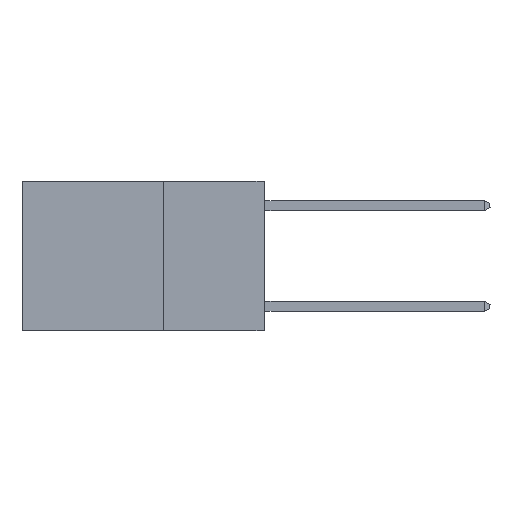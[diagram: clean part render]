
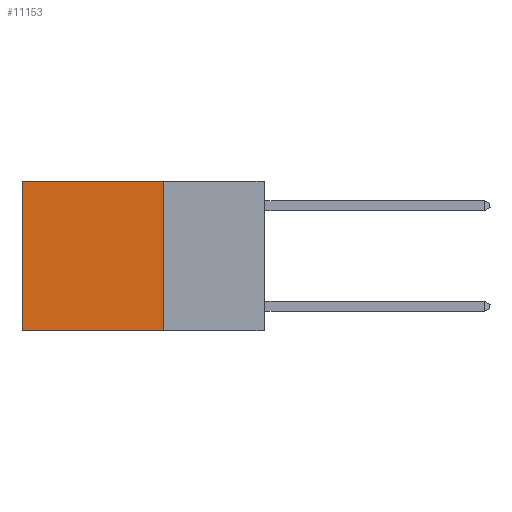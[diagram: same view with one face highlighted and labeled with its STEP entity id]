
A CAD part, left-side view. The second image highlights one B-rep face of the part: STEP entity #11153.
In plain terms, the highlighted planar face has unit normal (-1, 0, 0).
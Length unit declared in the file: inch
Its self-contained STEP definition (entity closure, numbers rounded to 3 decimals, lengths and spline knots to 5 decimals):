
#122 = CARTESIAN_POINT ( 'NONE',  ( 0.2625, 0.6, 0. ) ) ;
#252 = CARTESIAN_POINT ( 'NONE',  ( 0.2625, 0.25, -0.37 ) ) ;
#350 = EDGE_CURVE ( 'NONE', #2271, #13154, #4573, .T. ) ;
#555 = CARTESIAN_POINT ( 'NONE',  ( 0.2625, 0.25, 0. ) ) ;
#783 = ORIENTED_EDGE ( 'NONE', *, *, #350, .F. ) ;
#1790 = DIRECTION ( 'NONE',  ( 0., 1., 0. ) ) ;
#2104 = VERTEX_POINT ( 'NONE', #122 ) ;
#2271 = VERTEX_POINT ( 'NONE', #8878 ) ;
#2285 = ORIENTED_EDGE ( 'NONE', *, *, #7054, .F. ) ;
#3104 = CARTESIAN_POINT ( 'NONE',  ( 0.2625, 0.25, -0.37 ) ) ;
#3627 = DIRECTION ( 'NONE',  ( 0., 0., -1. ) ) ;
#4187 = VECTOR ( 'NONE', #1790, 39.37008 ) ;
#4573 = LINE ( 'NONE', #10926, #9846 ) ;
#4945 = VERTEX_POINT ( 'NONE', #7226 ) ;
#6442 = AXIS2_PLACEMENT_3D ( 'NONE', #13311, #10381, #10111 ) ;
#7054 = EDGE_CURVE ( 'NONE', #13154, #4945, #13433, .T. ) ;
#7226 = CARTESIAN_POINT ( 'NONE',  ( 0.2625, 0.6, -0.37 ) ) ;
#7231 = FACE_OUTER_BOUND ( 'NONE', #8491, .T. ) ;
#7802 = EDGE_CURVE ( 'NONE', #2271, #2104, #8914, .T. ) ;
#8491 = EDGE_LOOP ( 'NONE', ( #9115, #2285, #783, #10505 ) ) ;
#8859 = CARTESIAN_POINT ( 'NONE',  ( 0.2625, 0.6, 0. ) ) ;
#8878 = CARTESIAN_POINT ( 'NONE',  ( 0.2625, 0.25, 0. ) ) ;
#8914 = LINE ( 'NONE', #555, #12905 ) ;
#9109 = PLANE ( 'NONE',  #6442 ) ;
#9115 = ORIENTED_EDGE ( 'NONE', *, *, #12322, .T. ) ;
#9846 = VECTOR ( 'NONE', #13148, 39.37008 ) ;
#9919 = LINE ( 'NONE', #8859, #10047 ) ;
#10047 = VECTOR ( 'NONE', #3627, 39.37008 ) ;
#10111 = DIRECTION ( 'NONE',  ( 0., 0., -1. ) ) ;
#10381 = DIRECTION ( 'NONE',  ( 1., 0., 0. ) ) ;
#10505 = ORIENTED_EDGE ( 'NONE', *, *, #7802, .T. ) ;
#10926 = CARTESIAN_POINT ( 'NONE',  ( 0.2625, 0.25, 0. ) ) ;
#11153 = ADVANCED_FACE ( 'NONE', ( #7231 ), #9109, .F. ) ;
#12322 = EDGE_CURVE ( 'NONE', #2104, #4945, #9919, .T. ) ;
#12362 = DIRECTION ( 'NONE',  ( 0., 1., 0. ) ) ;
#12905 = VECTOR ( 'NONE', #12362, 39.37008 ) ;
#13148 = DIRECTION ( 'NONE',  ( 0., 0., -1. ) ) ;
#13154 = VERTEX_POINT ( 'NONE', #252 ) ;
#13311 = CARTESIAN_POINT ( 'NONE',  ( 0.2625, 0.25, 0. ) ) ;
#13433 = LINE ( 'NONE', #3104, #4187 ) ;
